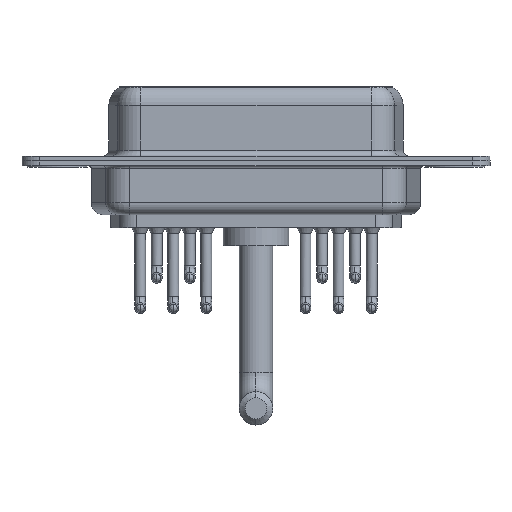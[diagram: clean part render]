
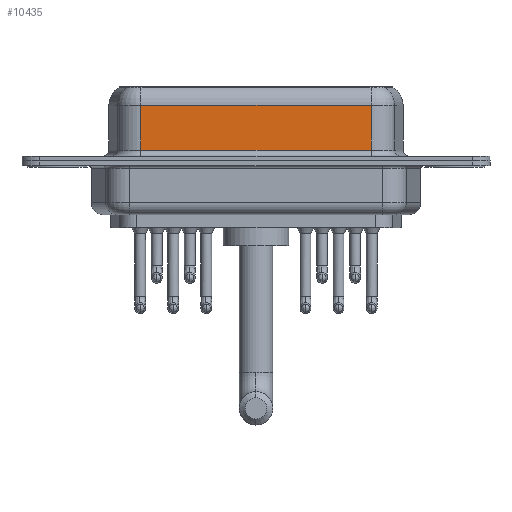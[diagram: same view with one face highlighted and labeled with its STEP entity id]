
A CAD part, front view. The second image highlights one B-rep face of the part: STEP entity #10435.
In plain terms, the highlighted planar face has unit normal (0, -1, 0).
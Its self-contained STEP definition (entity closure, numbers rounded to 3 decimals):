
#197 = CARTESIAN_POINT ( 'NONE',  ( 7.013, -3.95, 4.65 ) ) ;
#366 = CARTESIAN_POINT ( 'NONE',  ( 26.287, -3.95, 4.65 ) ) ;
#668 = VERTEX_POINT ( 'NONE', #2126 ) ;
#733 = VECTOR ( 'NONE', #10290, 1000. ) ;
#1053 = FACE_OUTER_BOUND ( 'NONE', #11972, .T. ) ;
#1312 = CARTESIAN_POINT ( 'NONE',  ( 26.287, -3.95, 0.9 ) ) ;
#1315 = DIRECTION ( 'NONE',  ( 0., 1., 0. ) ) ;
#1574 = VERTEX_POINT ( 'NONE', #3700 ) ;
#2126 = CARTESIAN_POINT ( 'NONE',  ( 7.013, -3.95, 0.9 ) ) ;
#2697 = DIRECTION ( 'NONE',  ( 0., 0., -1. ) ) ;
#3370 = EDGE_CURVE ( 'NONE', #10484, #1574, #16767, .T. ) ;
#3700 = CARTESIAN_POINT ( 'NONE',  ( 26.287, -3.95, 0.9 ) ) ;
#3809 = ORIENTED_EDGE ( 'NONE', *, *, #6964, .T. ) ;
#5045 = CARTESIAN_POINT ( 'NONE',  ( 26.287, -3.95, 6.4 ) ) ;
#5570 = DIRECTION ( 'NONE',  ( -1., 0., 0. ) ) ;
#6526 = DIRECTION ( 'NONE',  ( 1., 0., 0. ) ) ;
#6964 = EDGE_CURVE ( 'NONE', #13132, #668, #13146, .T. ) ;
#9213 = VECTOR ( 'NONE', #6526, 1000. ) ;
#9337 = EDGE_CURVE ( 'NONE', #668, #1574, #11662, .T. ) ;
#9459 = EDGE_CURVE ( 'NONE', #10484, #13132, #14713, .T. ) ;
#10031 = VECTOR ( 'NONE', #2697, 1000. ) ;
#10290 = DIRECTION ( 'NONE',  ( 0., 0., -1. ) ) ;
#10435 = ADVANCED_FACE ( 'NONE', ( #1053 ), #16691, .F. ) ;
#10484 = VERTEX_POINT ( 'NONE', #14380 ) ;
#11428 = AXIS2_PLACEMENT_3D ( 'NONE', #11494, #1315, #15586 ) ;
#11494 = CARTESIAN_POINT ( 'NONE',  ( 26.287, -3.95, 6.4 ) ) ;
#11662 = LINE ( 'NONE', #1312, #9213 ) ;
#11697 = CARTESIAN_POINT ( 'NONE',  ( 7.013, -3.95, 6.4 ) ) ;
#11972 = EDGE_LOOP ( 'NONE', ( #15464, #16653, #3809, #15678 ) ) ;
#13065 = VECTOR ( 'NONE', #5570, 1000. ) ;
#13132 = VERTEX_POINT ( 'NONE', #197 ) ;
#13146 = LINE ( 'NONE', #11697, #10031 ) ;
#14380 = CARTESIAN_POINT ( 'NONE',  ( 26.287, -3.95, 4.65 ) ) ;
#14713 = LINE ( 'NONE', #366, #13065 ) ;
#15464 = ORIENTED_EDGE ( 'NONE', *, *, #3370, .F. ) ;
#15586 = DIRECTION ( 'NONE',  ( 0., 0., 1. ) ) ;
#15678 = ORIENTED_EDGE ( 'NONE', *, *, #9337, .T. ) ;
#16653 = ORIENTED_EDGE ( 'NONE', *, *, #9459, .T. ) ;
#16691 = PLANE ( 'NONE',  #11428 ) ;
#16767 = LINE ( 'NONE', #5045, #733 ) ;
